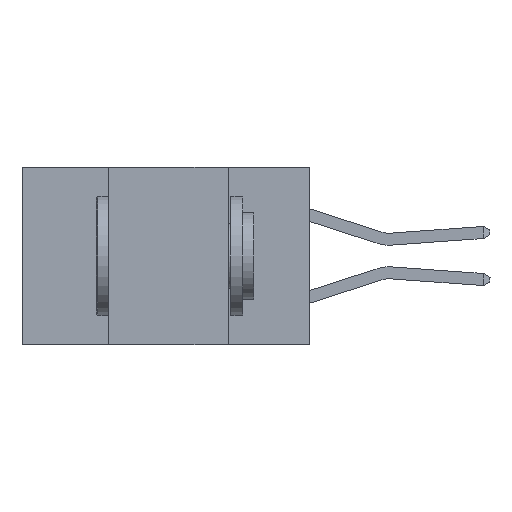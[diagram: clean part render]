
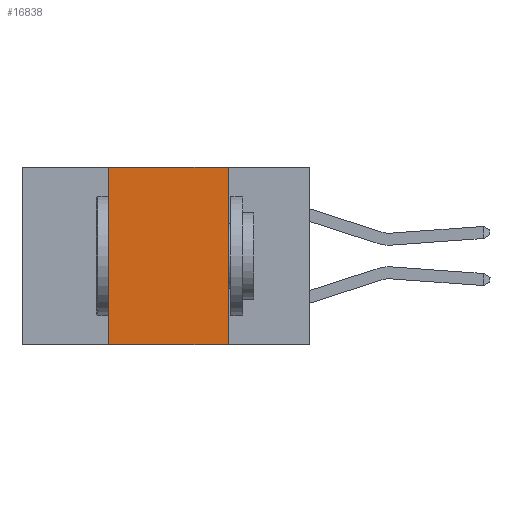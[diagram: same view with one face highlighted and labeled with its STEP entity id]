
A CAD part, left-side view. The second image highlights one B-rep face of the part: STEP entity #16838.
In plain terms, the highlighted planar face has unit normal (-1, 0, 0).
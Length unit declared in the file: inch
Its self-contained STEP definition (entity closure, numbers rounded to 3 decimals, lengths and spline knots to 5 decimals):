
#951 = VECTOR ( 'NONE', #18830, 39.37008 ) ;
#1153 = VECTOR ( 'NONE', #13375, 39.37008 ) ;
#2046 = CARTESIAN_POINT ( 'NONE',  ( 0., 0.6, -0.37 ) ) ;
#2286 = DIRECTION ( 'NONE',  ( 0., 0., 1. ) ) ;
#2650 = LINE ( 'NONE', #16716, #951 ) ;
#3556 = VERTEX_POINT ( 'NONE', #7319 ) ;
#4968 = VECTOR ( 'NONE', #2286, 39.37008 ) ;
#5445 = EDGE_CURVE ( 'NONE', #6129, #13323, #8591, .T. ) ;
#6129 = VERTEX_POINT ( 'NONE', #17471 ) ;
#7319 = CARTESIAN_POINT ( 'NONE',  ( 0., 0.17, -0.37 ) ) ;
#7642 = EDGE_CURVE ( 'NONE', #19358, #3556, #2650, .T. ) ;
#7879 = CARTESIAN_POINT ( 'NONE',  ( 0., 0.42, 0. ) ) ;
#8150 = DIRECTION ( 'NONE',  ( 1., 0., 0. ) ) ;
#8306 = DIRECTION ( 'NONE',  ( 0., 0., -1. ) ) ;
#8591 = LINE ( 'NONE', #22141, #4968 ) ;
#9770 = ORIENTED_EDGE ( 'NONE', *, *, #12307, .F. ) ;
#10284 = LINE ( 'NONE', #2046, #12801 ) ;
#10772 = ORIENTED_EDGE ( 'NONE', *, *, #22802, .T. ) ;
#12307 = EDGE_CURVE ( 'NONE', #13323, #19358, #12332, .T. ) ;
#12332 = LINE ( 'NONE', #15315, #1153 ) ;
#12801 = VECTOR ( 'NONE', #21809, 39.37008 ) ;
#12856 = EDGE_LOOP ( 'NONE', ( #15782, #9770, #16879, #10772 ) ) ;
#13323 = VERTEX_POINT ( 'NONE', #7879 ) ;
#13375 = DIRECTION ( 'NONE',  ( 0., -1., 0. ) ) ;
#13441 = PLANE ( 'NONE',  #14493 ) ;
#14493 = AXIS2_PLACEMENT_3D ( 'NONE', #18971, #8150, #8306 ) ;
#15315 = CARTESIAN_POINT ( 'NONE',  ( 0., 0.6, 0. ) ) ;
#15782 = ORIENTED_EDGE ( 'NONE', *, *, #7642, .F. ) ;
#16716 = CARTESIAN_POINT ( 'NONE',  ( 0., 0.17, 0. ) ) ;
#16838 = ADVANCED_FACE ( 'NONE', ( #22425 ), #13441, .F. ) ;
#16879 = ORIENTED_EDGE ( 'NONE', *, *, #5445, .F. ) ;
#17471 = CARTESIAN_POINT ( 'NONE',  ( 0., 0.42, -0.37 ) ) ;
#18718 = CARTESIAN_POINT ( 'NONE',  ( 0., 0.17, 0. ) ) ;
#18830 = DIRECTION ( 'NONE',  ( 0., 0., -1. ) ) ;
#18971 = CARTESIAN_POINT ( 'NONE',  ( 0., 0.6, 0. ) ) ;
#19358 = VERTEX_POINT ( 'NONE', #18718 ) ;
#21809 = DIRECTION ( 'NONE',  ( 0., -1., 0. ) ) ;
#22141 = CARTESIAN_POINT ( 'NONE',  ( 0., 0.42, 0. ) ) ;
#22425 = FACE_OUTER_BOUND ( 'NONE', #12856, .T. ) ;
#22802 = EDGE_CURVE ( 'NONE', #6129, #3556, #10284, .T. ) ;
